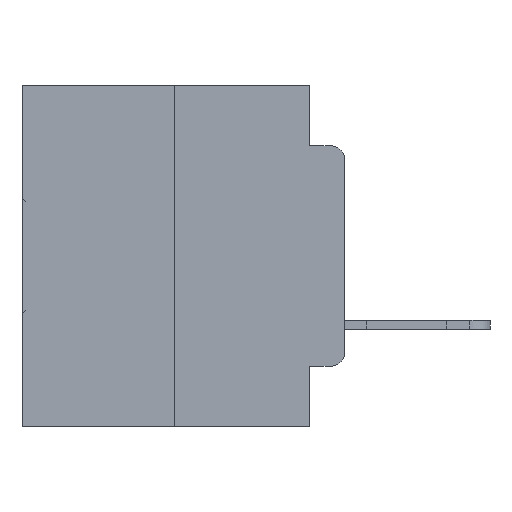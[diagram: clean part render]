
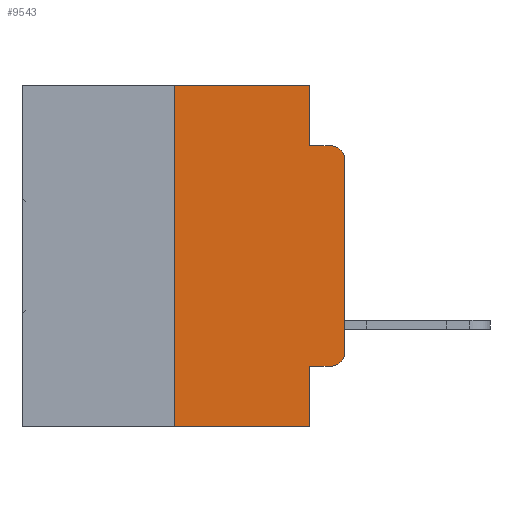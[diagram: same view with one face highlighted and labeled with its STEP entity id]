
A CAD part, left-side view. The second image highlights one B-rep face of the part: STEP entity #9543.
In plain terms, the highlighted planar face has unit normal (-1, 0, 0).
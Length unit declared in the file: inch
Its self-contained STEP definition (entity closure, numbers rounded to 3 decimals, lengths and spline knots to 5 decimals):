
#686 = EDGE_CURVE ( 'NONE', #3955, #17377, #30108, .T. ) ;
#922 = DIRECTION ( 'NONE',  ( 1., 0., 0. ) ) ;
#1042 = VECTOR ( 'NONE', #3020, 39.37008 ) ;
#1453 = VERTEX_POINT ( 'NONE', #17849 ) ;
#1538 = DIRECTION ( 'NONE',  ( 0., 0., 1. ) ) ;
#1630 = ORIENTED_EDGE ( 'NONE', *, *, #8858, .F. ) ;
#1751 = DIRECTION ( 'NONE',  ( 0., 0., 1. ) ) ;
#1814 = VERTEX_POINT ( 'NONE', #4955 ) ;
#1882 = CARTESIAN_POINT ( 'NONE',  ( 0., 0.02, -0.1085 ) ) ;
#1905 = LINE ( 'NONE', #25135, #1042 ) ;
#2082 = CARTESIAN_POINT ( 'NONE',  ( 0., 0.051, -0.4115 ) ) ;
#2388 = CARTESIAN_POINT ( 'NONE',  ( 0., 0., 0. ) ) ;
#3020 = DIRECTION ( 'NONE',  ( 0., -1., 0. ) ) ;
#3680 = EDGE_CURVE ( 'NONE', #17377, #1453, #28401, .T. ) ;
#3955 = VERTEX_POINT ( 'NONE', #27225 ) ;
#4472 = ORIENTED_EDGE ( 'NONE', *, *, #6105, .F. ) ;
#4608 = DIRECTION ( 'NONE',  ( 0., 0., -1. ) ) ;
#4937 = ORIENTED_EDGE ( 'NONE', *, *, #28897, .T. ) ;
#4955 = CARTESIAN_POINT ( 'NONE',  ( 0., 0.02, -0.0885 ) ) ;
#5966 = AXIS2_PLACEMENT_3D ( 'NONE', #1882, #19325, #4608 ) ;
#6105 = EDGE_CURVE ( 'NONE', #19920, #1814, #1905, .T. ) ;
#6536 = LINE ( 'NONE', #2082, #25201 ) ;
#6812 = CARTESIAN_POINT ( 'NONE',  ( 0., 0.473, -0.5 ) ) ;
#7733 = ORIENTED_EDGE ( 'NONE', *, *, #14363, .T. ) ;
#7856 = VERTEX_POINT ( 'NONE', #24435 ) ;
#7958 = CARTESIAN_POINT ( 'NONE',  ( 0., 0.473, 0. ) ) ;
#8356 = CARTESIAN_POINT ( 'NONE',  ( 0., 0.051, 0. ) ) ;
#8858 = EDGE_CURVE ( 'NONE', #23239, #19920, #26483, .T. ) ;
#8876 = ORIENTED_EDGE ( 'NONE', *, *, #21646, .F. ) ;
#9131 = VECTOR ( 'NONE', #1751, 39.37008 ) ;
#9412 = CARTESIAN_POINT ( 'NONE',  ( 0., 0.25, 0. ) ) ;
#9543 = ADVANCED_FACE ( 'NONE', ( #28296 ), #11226, .F. ) ;
#10407 = DIRECTION ( 'NONE',  ( 0., 0., -1. ) ) ;
#10524 = DIRECTION ( 'NONE',  ( -1., 0., 0. ) ) ;
#11226 = PLANE ( 'NONE',  #11874 ) ;
#11335 = ORIENTED_EDGE ( 'NONE', *, *, #686, .T. ) ;
#11433 = CARTESIAN_POINT ( 'NONE',  ( 0., 0.051, 0. ) ) ;
#11874 = AXIS2_PLACEMENT_3D ( 'NONE', #30472, #922, #18473 ) ;
#12082 = ORIENTED_EDGE ( 'NONE', *, *, #3680, .T. ) ;
#12250 = CARTESIAN_POINT ( 'NONE',  ( 0., 0.25, -0.5 ) ) ;
#12621 = CARTESIAN_POINT ( 'NONE',  ( 0., 0.25, 0. ) ) ;
#12880 = DIRECTION ( 'NONE',  ( 0., 0., -1. ) ) ;
#13171 = ORIENTED_EDGE ( 'NONE', *, *, #13790, .T. ) ;
#13790 = EDGE_CURVE ( 'NONE', #7856, #3955, #6536, .T. ) ;
#14363 = EDGE_CURVE ( 'NONE', #20811, #19031, #15646, .T. ) ;
#14963 = ORIENTED_EDGE ( 'NONE', *, *, #18086, .F. ) ;
#15646 = LINE ( 'NONE', #6812, #21347 ) ;
#16949 = VECTOR ( 'NONE', #1538, 39.37008 ) ;
#17301 = CARTESIAN_POINT ( 'NONE',  ( 0., 0.02, -0.3915 ) ) ;
#17377 = VERTEX_POINT ( 'NONE', #25641 ) ;
#17849 = CARTESIAN_POINT ( 'NONE',  ( 0., 0., -0.1085 ) ) ;
#18086 = EDGE_CURVE ( 'NONE', #7856, #19031, #21273, .T. ) ;
#18372 = CIRCLE ( 'NONE', #5966, 0.02 ) ;
#18473 = DIRECTION ( 'NONE',  ( 0., 0., -1. ) ) ;
#19031 = VERTEX_POINT ( 'NONE', #19695 ) ;
#19032 = AXIS2_PLACEMENT_3D ( 'NONE', #17301, #10524, #10407 ) ;
#19325 = DIRECTION ( 'NONE',  ( -1., 0., 0. ) ) ;
#19364 = ORIENTED_EDGE ( 'NONE', *, *, #23682, .F. ) ;
#19695 = CARTESIAN_POINT ( 'NONE',  ( 0., 0.051, -0.5 ) ) ;
#19920 = VERTEX_POINT ( 'NONE', #23726 ) ;
#20018 = VECTOR ( 'NONE', #20408, 39.37008 ) ;
#20408 = DIRECTION ( 'NONE',  ( 0., 0., -1. ) ) ;
#20811 = VERTEX_POINT ( 'NONE', #12250 ) ;
#20940 = LINE ( 'NONE', #7958, #26638 ) ;
#21273 = LINE ( 'NONE', #24932, #26955 ) ;
#21347 = VECTOR ( 'NONE', #21391, 39.37008 ) ;
#21391 = DIRECTION ( 'NONE',  ( 0., -1., 0. ) ) ;
#21646 = EDGE_CURVE ( 'NONE', #20811, #28225, #30519, .T. ) ;
#23239 = VERTEX_POINT ( 'NONE', #11433 ) ;
#23478 = EDGE_LOOP ( 'NONE', ( #12082, #4937, #4472, #1630, #19364, #8876, #7733, #14963, #13171, #11335 ) ) ;
#23682 = EDGE_CURVE ( 'NONE', #28225, #23239, #20940, .T. ) ;
#23726 = CARTESIAN_POINT ( 'NONE',  ( 0., 0.051, -0.0885 ) ) ;
#24435 = CARTESIAN_POINT ( 'NONE',  ( 0., 0.051, -0.4115 ) ) ;
#24932 = CARTESIAN_POINT ( 'NONE',  ( 0., 0.051, 0. ) ) ;
#25135 = CARTESIAN_POINT ( 'NONE',  ( 0., 0.051, -0.0885 ) ) ;
#25201 = VECTOR ( 'NONE', #29132, 39.37008 ) ;
#25641 = CARTESIAN_POINT ( 'NONE',  ( 0., 0., -0.3915 ) ) ;
#26483 = LINE ( 'NONE', #8356, #20018 ) ;
#26638 = VECTOR ( 'NONE', #27331, 39.37008 ) ;
#26955 = VECTOR ( 'NONE', #12880, 39.37008 ) ;
#27225 = CARTESIAN_POINT ( 'NONE',  ( 0., 0.02, -0.4115 ) ) ;
#27331 = DIRECTION ( 'NONE',  ( 0., -1., 0. ) ) ;
#28225 = VERTEX_POINT ( 'NONE', #12621 ) ;
#28296 = FACE_OUTER_BOUND ( 'NONE', #23478, .T. ) ;
#28401 = LINE ( 'NONE', #2388, #9131 ) ;
#28897 = EDGE_CURVE ( 'NONE', #1453, #1814, #18372, .T. ) ;
#29132 = DIRECTION ( 'NONE',  ( 0., -1., 0. ) ) ;
#30108 = CIRCLE ( 'NONE', #19032, 0.02 ) ;
#30472 = CARTESIAN_POINT ( 'NONE',  ( 0., 0.473, 0. ) ) ;
#30519 = LINE ( 'NONE', #9412, #16949 ) ;
